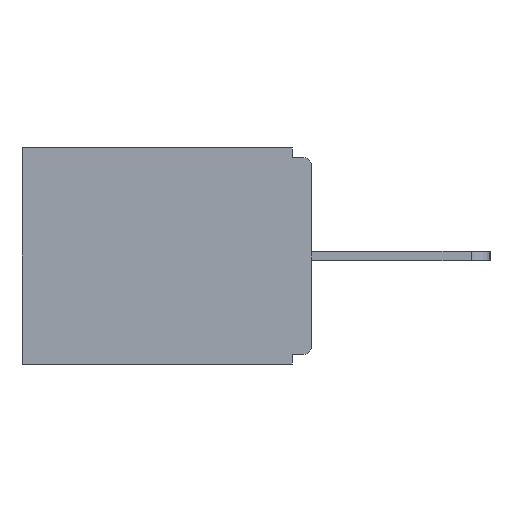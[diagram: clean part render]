
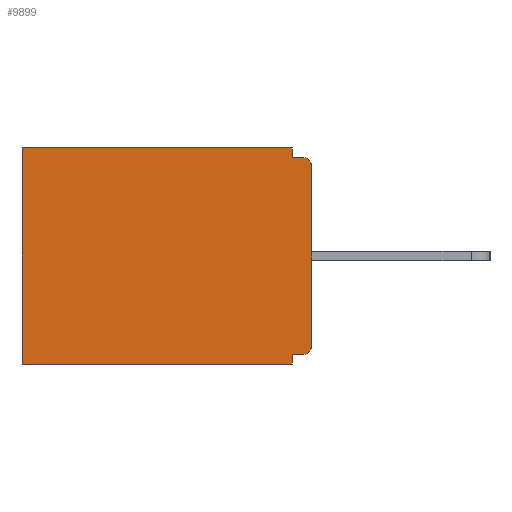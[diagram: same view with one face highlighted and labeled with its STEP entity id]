
A CAD part, left-side view. The second image highlights one B-rep face of the part: STEP entity #9899.
In plain terms, the highlighted planar face has unit normal (-1, 0, 0).
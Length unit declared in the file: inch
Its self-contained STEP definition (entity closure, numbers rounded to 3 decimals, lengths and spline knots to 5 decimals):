
#1151 = EDGE_CURVE ( 'NONE', #11902, #6007, #19109, .T. ) ;
#1213 = LINE ( 'NONE', #22787, #25148 ) ;
#1335 = DIRECTION ( 'NONE',  ( 0., 0., -1. ) ) ;
#2666 = EDGE_LOOP ( 'NONE', ( #5047, #21073, #15236, #23861, #11753, #25249, #11537, #13186, #16944, #4507 ) ) ;
#2802 = VECTOR ( 'NONE', #4774, 39.37008 ) ;
#2901 = VERTEX_POINT ( 'NONE', #11878 ) ;
#2933 = CIRCLE ( 'NONE', #13178, 0.015 ) ;
#3187 = LINE ( 'NONE', #7037, #9703 ) ;
#3998 = EDGE_CURVE ( 'NONE', #2901, #18953, #24359, .T. ) ;
#4507 = ORIENTED_EDGE ( 'NONE', *, *, #6989, .F. ) ;
#4716 = DIRECTION ( 'NONE',  ( 0., -1., 0. ) ) ;
#4774 = DIRECTION ( 'NONE',  ( 0., 0., -1. ) ) ;
#4827 = CARTESIAN_POINT ( 'NONE',  ( 0.298, 0.015, -0.03 ) ) ;
#4855 = EDGE_CURVE ( 'NONE', #6007, #9412, #7222, .T. ) ;
#5029 = CARTESIAN_POINT ( 'NONE',  ( 0.298, 0., 0. ) ) ;
#5047 = ORIENTED_EDGE ( 'NONE', *, *, #3998, .T. ) ;
#5630 = CARTESIAN_POINT ( 'NONE',  ( 0.298, 0.031, 0. ) ) ;
#6007 = VERTEX_POINT ( 'NONE', #18014 ) ;
#6989 = EDGE_CURVE ( 'NONE', #2901, #8535, #20481, .T. ) ;
#7037 = CARTESIAN_POINT ( 'NONE',  ( 0.298, 0., -0.015 ) ) ;
#7222 = LINE ( 'NONE', #16850, #2802 ) ;
#7397 = VECTOR ( 'NONE', #11690, 39.37008 ) ;
#8105 = CARTESIAN_POINT ( 'NONE',  ( 0.298, 0.015, -0.015 ) ) ;
#8535 = VERTEX_POINT ( 'NONE', #15848 ) ;
#8661 = EDGE_CURVE ( 'NONE', #19129, #20719, #20065, .T. ) ;
#8905 = CARTESIAN_POINT ( 'NONE',  ( 0.298, 0.46, -0.343 ) ) ;
#9048 = CARTESIAN_POINT ( 'NONE',  ( 0.298, 0.015, -0.313 ) ) ;
#9224 = DIRECTION ( 'NONE',  ( 0., 1., 0. ) ) ;
#9337 = VECTOR ( 'NONE', #14193, 39.37008 ) ;
#9412 = VERTEX_POINT ( 'NONE', #24594 ) ;
#9703 = VECTOR ( 'NONE', #4716, 39.37008 ) ;
#9899 = ADVANCED_FACE ( 'NONE', ( #11199 ), #11329, .F. ) ;
#10138 = LINE ( 'NONE', #13616, #7397 ) ;
#10303 = CARTESIAN_POINT ( 'NONE',  ( 0.298, 0., 0. ) ) ;
#10445 = EDGE_CURVE ( 'NONE', #11902, #8535, #2933, .T. ) ;
#11199 = FACE_OUTER_BOUND ( 'NONE', #2666, .T. ) ;
#11329 = PLANE ( 'NONE',  #14796 ) ;
#11510 = DIRECTION ( 'NONE',  ( 0., 1., 0. ) ) ;
#11537 = ORIENTED_EDGE ( 'NONE', *, *, #4855, .F. ) ;
#11690 = DIRECTION ( 'NONE',  ( 0., 0., -1. ) ) ;
#11753 = ORIENTED_EDGE ( 'NONE', *, *, #16521, .T. ) ;
#11878 = CARTESIAN_POINT ( 'NONE',  ( 0.298, 0., -0.03 ) ) ;
#11902 = VERTEX_POINT ( 'NONE', #18777 ) ;
#12883 = DIRECTION ( 'NONE',  ( 0., 0., -1. ) ) ;
#13178 = AXIS2_PLACEMENT_3D ( 'NONE', #9048, #24711, #1335 ) ;
#13186 = ORIENTED_EDGE ( 'NONE', *, *, #1151, .F. ) ;
#13616 = CARTESIAN_POINT ( 'NONE',  ( 0.298, 0.46, 0. ) ) ;
#14193 = DIRECTION ( 'NONE',  ( 0., 0., -1. ) ) ;
#14446 = CARTESIAN_POINT ( 'NONE',  ( 0.298, 0., 0. ) ) ;
#14796 = AXIS2_PLACEMENT_3D ( 'NONE', #5029, #25082, #12883 ) ;
#15122 = DIRECTION ( 'NONE',  ( 0., 0., -1. ) ) ;
#15236 = ORIENTED_EDGE ( 'NONE', *, *, #18196, .F. ) ;
#15848 = CARTESIAN_POINT ( 'NONE',  ( 0.298, 0., -0.313 ) ) ;
#15954 = CARTESIAN_POINT ( 'NONE',  ( 0.298, 0.031, -0.015 ) ) ;
#16226 = DIRECTION ( 'NONE',  ( 0., 1., 0. ) ) ;
#16521 = EDGE_CURVE ( 'NONE', #20719, #23645, #10138, .T. ) ;
#16850 = CARTESIAN_POINT ( 'NONE',  ( 0.298, 0.031, -0.343 ) ) ;
#16944 = ORIENTED_EDGE ( 'NONE', *, *, #10445, .T. ) ;
#17060 = CARTESIAN_POINT ( 'NONE',  ( 0.298, 0., -0.328 ) ) ;
#17195 = VECTOR ( 'NONE', #16226, 39.37008 ) ;
#17547 = CARTESIAN_POINT ( 'NONE',  ( 0.298, 0., -0.343 ) ) ;
#18014 = CARTESIAN_POINT ( 'NONE',  ( 0.298, 0.031, -0.328 ) ) ;
#18196 = EDGE_CURVE ( 'NONE', #19129, #23132, #1213, .T. ) ;
#18777 = CARTESIAN_POINT ( 'NONE',  ( 0.298, 0.015, -0.328 ) ) ;
#18953 = VERTEX_POINT ( 'NONE', #8105 ) ;
#19109 = LINE ( 'NONE', #17060, #20182 ) ;
#19129 = VERTEX_POINT ( 'NONE', #5630 ) ;
#20065 = LINE ( 'NONE', #10303, #17195 ) ;
#20182 = VECTOR ( 'NONE', #9224, 39.37008 ) ;
#20481 = LINE ( 'NONE', #14446, #9337 ) ;
#20719 = VERTEX_POINT ( 'NONE', #21031 ) ;
#20773 = DIRECTION ( 'NONE',  ( -1., 0., 0. ) ) ;
#20864 = EDGE_CURVE ( 'NONE', #9412, #23645, #23332, .T. ) ;
#21031 = CARTESIAN_POINT ( 'NONE',  ( 0.298, 0.46, 0. ) ) ;
#21073 = ORIENTED_EDGE ( 'NONE', *, *, #21958, .F. ) ;
#21085 = AXIS2_PLACEMENT_3D ( 'NONE', #4827, #20773, #15122 ) ;
#21956 = VECTOR ( 'NONE', #11510, 39.37008 ) ;
#21958 = EDGE_CURVE ( 'NONE', #23132, #18953, #3187, .T. ) ;
#22787 = CARTESIAN_POINT ( 'NONE',  ( 0.298, 0.031, -0.343 ) ) ;
#23132 = VERTEX_POINT ( 'NONE', #15954 ) ;
#23332 = LINE ( 'NONE', #17547, #21956 ) ;
#23645 = VERTEX_POINT ( 'NONE', #8905 ) ;
#23861 = ORIENTED_EDGE ( 'NONE', *, *, #8661, .T. ) ;
#24359 = CIRCLE ( 'NONE', #21085, 0.015 ) ;
#24594 = CARTESIAN_POINT ( 'NONE',  ( 0.298, 0.031, -0.343 ) ) ;
#24711 = DIRECTION ( 'NONE',  ( -1., 0., 0. ) ) ;
#25082 = DIRECTION ( 'NONE',  ( 1., 0., 0. ) ) ;
#25100 = DIRECTION ( 'NONE',  ( 0., 0., -1. ) ) ;
#25148 = VECTOR ( 'NONE', #25100, 39.37008 ) ;
#25249 = ORIENTED_EDGE ( 'NONE', *, *, #20864, .F. ) ;
